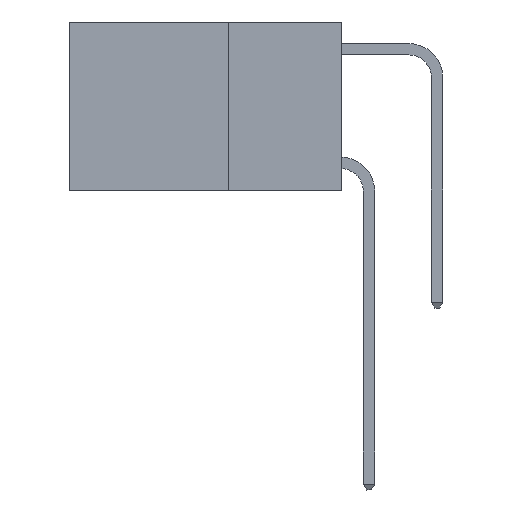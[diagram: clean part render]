
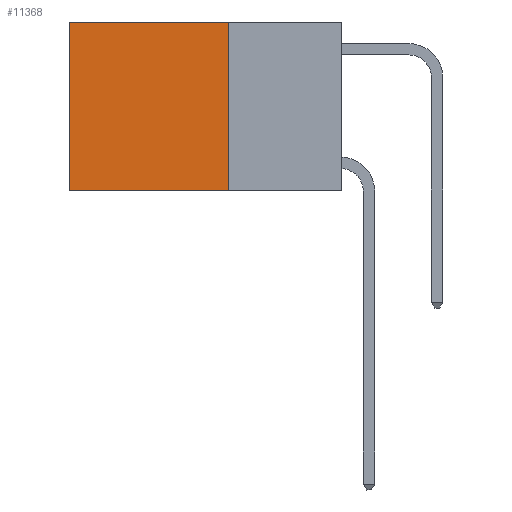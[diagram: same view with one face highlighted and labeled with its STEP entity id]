
A CAD part, left-side view. The second image highlights one B-rep face of the part: STEP entity #11368.
In plain terms, the highlighted planar face has unit normal (-1, 0, 0).
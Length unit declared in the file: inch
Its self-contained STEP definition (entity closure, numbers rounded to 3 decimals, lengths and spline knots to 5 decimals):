
#234 = CARTESIAN_POINT ( 'NONE',  ( 0.2625, 0.25, 0. ) ) ;
#343 = DIRECTION ( 'NONE',  ( 0., 0., -1. ) ) ;
#406 = CARTESIAN_POINT ( 'NONE',  ( 0.2625, 0.25, 0. ) ) ;
#461 = EDGE_CURVE ( 'NONE', #10992, #5629, #1196, .T. ) ;
#548 = ORIENTED_EDGE ( 'NONE', *, *, #5823, .F. ) ;
#1196 = LINE ( 'NONE', #234, #8795 ) ;
#1272 = DIRECTION ( 'NONE',  ( 1., 0., 0. ) ) ;
#2368 = ORIENTED_EDGE ( 'NONE', *, *, #9433, .F. ) ;
#2943 = AXIS2_PLACEMENT_3D ( 'NONE', #406, #1272, #343 ) ;
#2984 = LINE ( 'NONE', #4817, #11865 ) ;
#3512 = CARTESIAN_POINT ( 'NONE',  ( 0.2625, 0.25, 0. ) ) ;
#3683 = DIRECTION ( 'NONE',  ( 0., 0., -1. ) ) ;
#3733 = VECTOR ( 'NONE', #3683, 39.37008 ) ;
#3871 = DIRECTION ( 'NONE',  ( 0., 1., 0. ) ) ;
#4047 = CARTESIAN_POINT ( 'NONE',  ( 0.2625, 0.25, -0.37 ) ) ;
#4051 = CARTESIAN_POINT ( 'NONE',  ( 0.2625, 0.6, 0. ) ) ;
#4302 = CARTESIAN_POINT ( 'NONE',  ( 0.2625, 0.6, 0. ) ) ;
#4817 = CARTESIAN_POINT ( 'NONE',  ( 0.2625, 0.25, -0.37 ) ) ;
#5540 = VERTEX_POINT ( 'NONE', #4047 ) ;
#5629 = VERTEX_POINT ( 'NONE', #4302 ) ;
#5823 = EDGE_CURVE ( 'NONE', #10992, #5540, #9336, .T. ) ;
#6008 = PLANE ( 'NONE',  #2943 ) ;
#7260 = CARTESIAN_POINT ( 'NONE',  ( 0.2625, 0.25, 0. ) ) ;
#8072 = EDGE_LOOP ( 'NONE', ( #9503, #2368, #548, #9527 ) ) ;
#8344 = VECTOR ( 'NONE', #10470, 39.37008 ) ;
#8795 = VECTOR ( 'NONE', #11217, 39.37008 ) ;
#9173 = CARTESIAN_POINT ( 'NONE',  ( 0.2625, 0.6, -0.37 ) ) ;
#9336 = LINE ( 'NONE', #7260, #3733 ) ;
#9433 = EDGE_CURVE ( 'NONE', #5540, #10604, #2984, .T. ) ;
#9503 = ORIENTED_EDGE ( 'NONE', *, *, #10849, .T. ) ;
#9527 = ORIENTED_EDGE ( 'NONE', *, *, #461, .T. ) ;
#10470 = DIRECTION ( 'NONE',  ( 0., 0., -1. ) ) ;
#10604 = VERTEX_POINT ( 'NONE', #9173 ) ;
#10635 = FACE_OUTER_BOUND ( 'NONE', #8072, .T. ) ;
#10654 = LINE ( 'NONE', #4051, #8344 ) ;
#10849 = EDGE_CURVE ( 'NONE', #5629, #10604, #10654, .T. ) ;
#10992 = VERTEX_POINT ( 'NONE', #3512 ) ;
#11217 = DIRECTION ( 'NONE',  ( 0., 1., 0. ) ) ;
#11368 = ADVANCED_FACE ( 'NONE', ( #10635 ), #6008, .F. ) ;
#11865 = VECTOR ( 'NONE', #3871, 39.37008 ) ;
